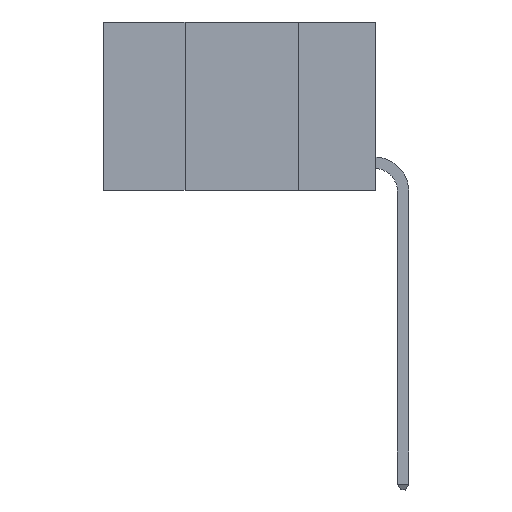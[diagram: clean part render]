
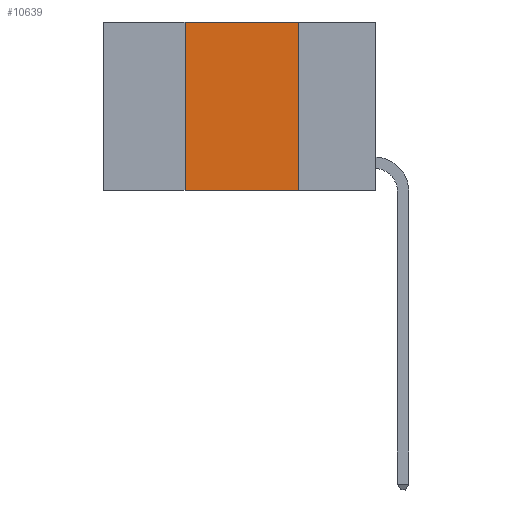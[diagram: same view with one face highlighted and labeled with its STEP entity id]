
A CAD part, left-side view. The second image highlights one B-rep face of the part: STEP entity #10639.
In plain terms, the highlighted planar face has unit normal (-1, 0, 0).
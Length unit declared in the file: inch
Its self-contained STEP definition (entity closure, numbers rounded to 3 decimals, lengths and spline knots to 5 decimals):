
#3491 = EDGE_CURVE ( 'NONE', #5369, #15416, #4154, .T. ) ;
#3790 = DIRECTION ( 'NONE',  ( 1., 0., 0. ) ) ;
#3983 = LINE ( 'NONE', #20157, #8743 ) ;
#4154 = LINE ( 'NONE', #21590, #19454 ) ;
#4199 = CARTESIAN_POINT ( 'NONE',  ( 0., 0.17, 0. ) ) ;
#5362 = DIRECTION ( 'NONE',  ( 0., -1., 0. ) ) ;
#5369 = VERTEX_POINT ( 'NONE', #7750 ) ;
#5697 = DIRECTION ( 'NONE',  ( 0., -1., 0. ) ) ;
#5835 = AXIS2_PLACEMENT_3D ( 'NONE', #25646, #3790, #17792 ) ;
#6542 = EDGE_LOOP ( 'NONE', ( #18480, #22488, #11040, #15388 ) ) ;
#6650 = CARTESIAN_POINT ( 'NONE',  ( 0., 0.17, -0.37 ) ) ;
#7409 = CARTESIAN_POINT ( 'NONE',  ( 0., 0.6, -0.37 ) ) ;
#7734 = VERTEX_POINT ( 'NONE', #17407 ) ;
#7750 = CARTESIAN_POINT ( 'NONE',  ( 0., 0.42, 0. ) ) ;
#8743 = VECTOR ( 'NONE', #22159, 39.37008 ) ;
#9405 = VECTOR ( 'NONE', #5362, 39.37008 ) ;
#9511 = VECTOR ( 'NONE', #23134, 39.37008 ) ;
#10471 = EDGE_CURVE ( 'NONE', #7734, #5369, #14758, .T. ) ;
#10639 = ADVANCED_FACE ( 'NONE', ( #20962 ), #21658, .F. ) ;
#11040 = ORIENTED_EDGE ( 'NONE', *, *, #10471, .F. ) ;
#13290 = EDGE_CURVE ( 'NONE', #7734, #25558, #25187, .T. ) ;
#14758 = LINE ( 'NONE', #15180, #9511 ) ;
#15180 = CARTESIAN_POINT ( 'NONE',  ( 0., 0.42, 0. ) ) ;
#15388 = ORIENTED_EDGE ( 'NONE', *, *, #13290, .T. ) ;
#15416 = VERTEX_POINT ( 'NONE', #4199 ) ;
#17407 = CARTESIAN_POINT ( 'NONE',  ( 0., 0.42, -0.37 ) ) ;
#17792 = DIRECTION ( 'NONE',  ( 0., 0., -1. ) ) ;
#18480 = ORIENTED_EDGE ( 'NONE', *, *, #24231, .F. ) ;
#19454 = VECTOR ( 'NONE', #5697, 39.37008 ) ;
#20157 = CARTESIAN_POINT ( 'NONE',  ( 0., 0.17, 0. ) ) ;
#20962 = FACE_OUTER_BOUND ( 'NONE', #6542, .T. ) ;
#21590 = CARTESIAN_POINT ( 'NONE',  ( 0., 0.6, 0. ) ) ;
#21658 = PLANE ( 'NONE',  #5835 ) ;
#22159 = DIRECTION ( 'NONE',  ( 0., 0., -1. ) ) ;
#22488 = ORIENTED_EDGE ( 'NONE', *, *, #3491, .F. ) ;
#23134 = DIRECTION ( 'NONE',  ( 0., 0., 1. ) ) ;
#24231 = EDGE_CURVE ( 'NONE', #15416, #25558, #3983, .T. ) ;
#25187 = LINE ( 'NONE', #7409, #9405 ) ;
#25558 = VERTEX_POINT ( 'NONE', #6650 ) ;
#25646 = CARTESIAN_POINT ( 'NONE',  ( 0., 0.6, 0. ) ) ;
